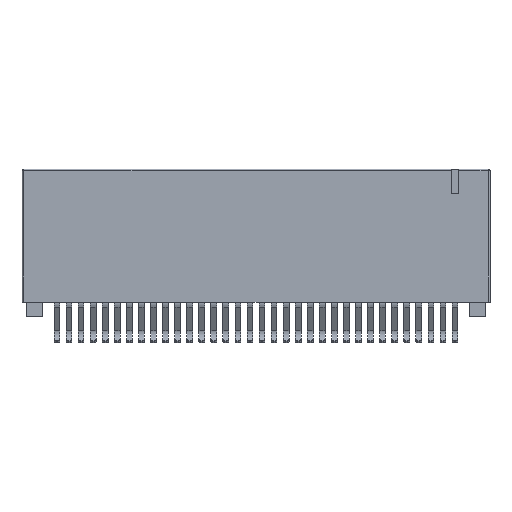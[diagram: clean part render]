
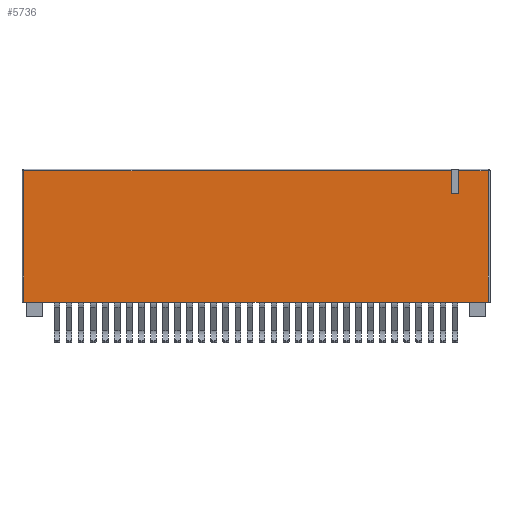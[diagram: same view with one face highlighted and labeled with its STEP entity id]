
A CAD part, top view. The second image highlights one B-rep face of the part: STEP entity #5736.
In plain terms, the highlighted planar face has unit normal (0, 0, 1).
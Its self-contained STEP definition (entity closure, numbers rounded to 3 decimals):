
#1791 = CARTESIAN_POINT ( 'NONE',  ( 0.2, 15.5, 0. ) ) ;
#3467 = VECTOR ( 'NONE', #11895, 1000. ) ;
#3570 = LINE ( 'NONE', #11496, #3467 ) ;
#4228 = CARTESIAN_POINT ( 'NONE',  ( 0.2, 1.5, 0. ) ) ;
#5489 = FACE_OUTER_BOUND ( 'NONE', #25807, .T. ) ;
#5736 = ADVANCED_FACE ( 'NONE', ( #5489 ), #7407, .F. ) ;
#5757 = DIRECTION ( 'NONE',  ( 0., 0., -1. ) ) ;
#5759 = LINE ( 'NONE', #1791, #10748 ) ;
#5921 = AXIS2_PLACEMENT_3D ( 'NONE', #24062, #5757, #17901 ) ;
#5965 = ORIENTED_EDGE ( 'NONE', *, *, #25978, .T. ) ;
#7056 = DIRECTION ( 'NONE',  ( 0., 1., 0. ) ) ;
#7357 = CARTESIAN_POINT ( 'NONE',  ( 45.205, 12.95, 0. ) ) ;
#7407 = PLANE ( 'NONE',  #5921 ) ;
#7678 = VECTOR ( 'NONE', #7056, 1000. ) ;
#7695 = LINE ( 'NONE', #23704, #14196 ) ;
#8075 = DIRECTION ( 'NONE',  ( 0., -1., 0. ) ) ;
#8246 = ORIENTED_EDGE ( 'NONE', *, *, #22514, .T. ) ;
#8962 = DIRECTION ( 'NONE',  ( -1., 0., 0. ) ) ;
#9324 = ORIENTED_EDGE ( 'NONE', *, *, #9870, .T. ) ;
#9819 = VERTEX_POINT ( 'NONE', #26369 ) ;
#9870 = EDGE_CURVE ( 'NONE', #18269, #10558, #5759, .T. ) ;
#10558 = VERTEX_POINT ( 'NONE', #4228 ) ;
#10748 = VECTOR ( 'NONE', #8075, 1000. ) ;
#10961 = EDGE_CURVE ( 'NONE', #12398, #18269, #24523, .T. ) ;
#11316 = DIRECTION ( 'NONE',  ( 0., 1., 0. ) ) ;
#11496 = CARTESIAN_POINT ( 'NONE',  ( 45.205, 12.95, 0. ) ) ;
#11595 = VERTEX_POINT ( 'NONE', #22122 ) ;
#11895 = DIRECTION ( 'NONE',  ( 1., 0., 0. ) ) ;
#12398 = VERTEX_POINT ( 'NONE', #17533 ) ;
#13383 = ORIENTED_EDGE ( 'NONE', *, *, #15204, .F. ) ;
#13591 = CARTESIAN_POINT ( 'NONE',  ( 49.28, 1.5, 0. ) ) ;
#13644 = ORIENTED_EDGE ( 'NONE', *, *, #24361, .F. ) ;
#14196 = VECTOR ( 'NONE', #18046, 1000. ) ;
#14569 = CARTESIAN_POINT ( 'NONE',  ( 45.205, 12.95, 0. ) ) ;
#15204 = EDGE_CURVE ( 'NONE', #26855, #16068, #3570, .T. ) ;
#15438 = VECTOR ( 'NONE', #11316, 1000. ) ;
#15650 = CARTESIAN_POINT ( 'NONE',  ( 45.985, 12.95, 0. ) ) ;
#16068 = VERTEX_POINT ( 'NONE', #24002 ) ;
#16567 = VECTOR ( 'NONE', #8962, 1000. ) ;
#16670 = CARTESIAN_POINT ( 'NONE',  ( 49.08, 15.5, 0. ) ) ;
#16786 = ORIENTED_EDGE ( 'NONE', *, *, #25837, .T. ) ;
#17185 = LINE ( 'NONE', #7357, #15438 ) ;
#17533 = CARTESIAN_POINT ( 'NONE',  ( 45.205, 15.3, 0. ) ) ;
#17901 = DIRECTION ( 'NONE',  ( -1., 0., 0. ) ) ;
#18046 = DIRECTION ( 'NONE',  ( -1., 0., 0. ) ) ;
#18176 = VERTEX_POINT ( 'NONE', #21693 ) ;
#18269 = VERTEX_POINT ( 'NONE', #22491 ) ;
#18670 = EDGE_CURVE ( 'NONE', #11595, #10558, #21790, .T. ) ;
#20923 = LINE ( 'NONE', #16670, #22476 ) ;
#20983 = ORIENTED_EDGE ( 'NONE', *, *, #18670, .F. ) ;
#21383 = ORIENTED_EDGE ( 'NONE', *, *, #10961, .T. ) ;
#21693 = CARTESIAN_POINT ( 'NONE',  ( 45.985, 15.3, 0. ) ) ;
#21790 = LINE ( 'NONE', #13591, #16567 ) ;
#22122 = CARTESIAN_POINT ( 'NONE',  ( 49.08, 1.5, 0. ) ) ;
#22476 = VECTOR ( 'NONE', #25009, 1000. ) ;
#22491 = CARTESIAN_POINT ( 'NONE',  ( 0.2, 15.3, 0. ) ) ;
#22514 = EDGE_CURVE ( 'NONE', #26855, #12398, #17185, .T. ) ;
#23704 = CARTESIAN_POINT ( 'NONE',  ( 0., 15.3, 0. ) ) ;
#24002 = CARTESIAN_POINT ( 'NONE',  ( 45.985, 12.95, 0. ) ) ;
#24062 = CARTESIAN_POINT ( 'NONE',  ( 0., 15.5, 0. ) ) ;
#24266 = CARTESIAN_POINT ( 'NONE',  ( 0., 15.3, 0. ) ) ;
#24361 = EDGE_CURVE ( 'NONE', #16068, #18176, #26030, .T. ) ;
#24523 = LINE ( 'NONE', #24266, #26837 ) ;
#25009 = DIRECTION ( 'NONE',  ( 0., 1., 0. ) ) ;
#25807 = EDGE_LOOP ( 'NONE', ( #13383, #8246, #21383, #9324, #20983, #5965, #16786, #13644 ) ) ;
#25837 = EDGE_CURVE ( 'NONE', #9819, #18176, #7695, .T. ) ;
#25978 = EDGE_CURVE ( 'NONE', #11595, #9819, #20923, .T. ) ;
#26030 = LINE ( 'NONE', #15650, #7678 ) ;
#26369 = CARTESIAN_POINT ( 'NONE',  ( 49.08, 15.3, 0. ) ) ;
#26706 = DIRECTION ( 'NONE',  ( -1., 0., 0. ) ) ;
#26837 = VECTOR ( 'NONE', #26706, 1000. ) ;
#26855 = VERTEX_POINT ( 'NONE', #14569 ) ;
